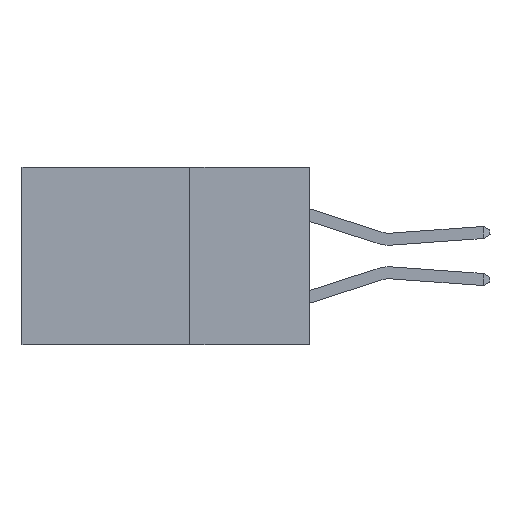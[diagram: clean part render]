
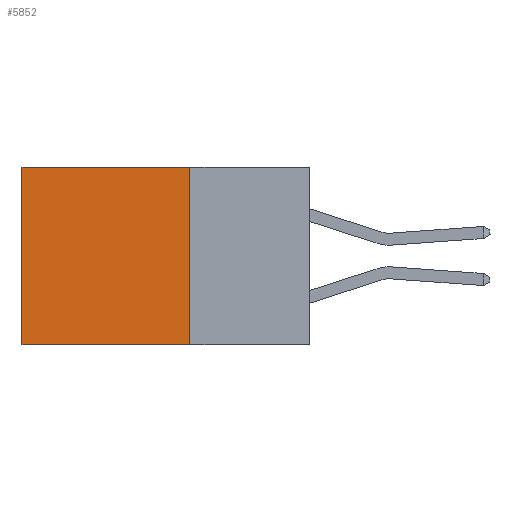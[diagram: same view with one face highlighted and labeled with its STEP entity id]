
A CAD part, left-side view. The second image highlights one B-rep face of the part: STEP entity #5852.
In plain terms, the highlighted planar face has unit normal (-1, 0, 0).
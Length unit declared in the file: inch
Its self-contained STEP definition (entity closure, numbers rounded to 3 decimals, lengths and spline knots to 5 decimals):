
#193 = LINE ( 'NONE', #22094, #25276 ) ;
#401 = VECTOR ( 'NONE', #10809, 39.37008 ) ;
#3036 = VERTEX_POINT ( 'NONE', #13777 ) ;
#3529 = CARTESIAN_POINT ( 'NONE',  ( 0.298, 0.25, 0. ) ) ;
#4876 = ORIENTED_EDGE ( 'NONE', *, *, #19787, .F. ) ;
#4877 = ORIENTED_EDGE ( 'NONE', *, *, #13368, .F. ) ;
#4901 = VECTOR ( 'NONE', #12594, 39.37008 ) ;
#5393 = ORIENTED_EDGE ( 'NONE', *, *, #18111, .T. ) ;
#5852 = ADVANCED_FACE ( 'NONE', ( #11360 ), #16904, .F. ) ;
#6767 = CARTESIAN_POINT ( 'NONE',  ( 0.298, 0.6, -0.37 ) ) ;
#6878 = LINE ( 'NONE', #18078, #401 ) ;
#7894 = VERTEX_POINT ( 'NONE', #9087 ) ;
#8476 = LINE ( 'NONE', #3529, #26319 ) ;
#9087 = CARTESIAN_POINT ( 'NONE',  ( 0.298, 0.25, -0.37 ) ) ;
#10809 = DIRECTION ( 'NONE',  ( 0., 0., -1. ) ) ;
#11151 = ORIENTED_EDGE ( 'NONE', *, *, #16788, .T. ) ;
#11360 = FACE_OUTER_BOUND ( 'NONE', #30396, .T. ) ;
#12594 = DIRECTION ( 'NONE',  ( 0., 0., -1. ) ) ;
#13368 = EDGE_CURVE ( 'NONE', #14606, #7894, #23509, .T. ) ;
#13777 = CARTESIAN_POINT ( 'NONE',  ( 0.298, 0.6, 0. ) ) ;
#14606 = VERTEX_POINT ( 'NONE', #28596 ) ;
#15042 = CARTESIAN_POINT ( 'NONE',  ( 0.298, 0.25, 0. ) ) ;
#16788 = EDGE_CURVE ( 'NONE', #14606, #3036, #8476, .T. ) ;
#16864 = CARTESIAN_POINT ( 'NONE',  ( 0.298, 0.25, 0. ) ) ;
#16904 = PLANE ( 'NONE',  #20498 ) ;
#18078 = CARTESIAN_POINT ( 'NONE',  ( 0.298, 0.6, 0. ) ) ;
#18111 = EDGE_CURVE ( 'NONE', #3036, #30561, #6878, .T. ) ;
#18155 = DIRECTION ( 'NONE',  ( 0., 1., 0. ) ) ;
#19685 = DIRECTION ( 'NONE',  ( 0., 1., 0. ) ) ;
#19787 = EDGE_CURVE ( 'NONE', #7894, #30561, #193, .T. ) ;
#20429 = DIRECTION ( 'NONE',  ( 0., 0., -1. ) ) ;
#20498 = AXIS2_PLACEMENT_3D ( 'NONE', #16864, #20505, #20429 ) ;
#20505 = DIRECTION ( 'NONE',  ( 1., 0., 0. ) ) ;
#22094 = CARTESIAN_POINT ( 'NONE',  ( 0.298, 0.25, -0.37 ) ) ;
#23509 = LINE ( 'NONE', #15042, #4901 ) ;
#25276 = VECTOR ( 'NONE', #19685, 39.37008 ) ;
#26319 = VECTOR ( 'NONE', #18155, 39.37008 ) ;
#28596 = CARTESIAN_POINT ( 'NONE',  ( 0.298, 0.25, 0. ) ) ;
#30396 = EDGE_LOOP ( 'NONE', ( #5393, #4876, #4877, #11151 ) ) ;
#30561 = VERTEX_POINT ( 'NONE', #6767 ) ;
